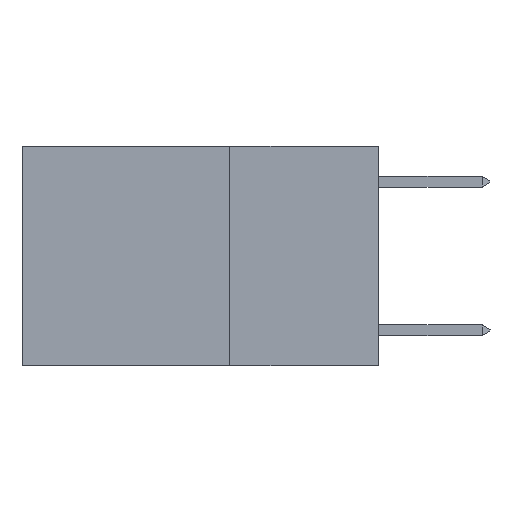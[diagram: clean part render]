
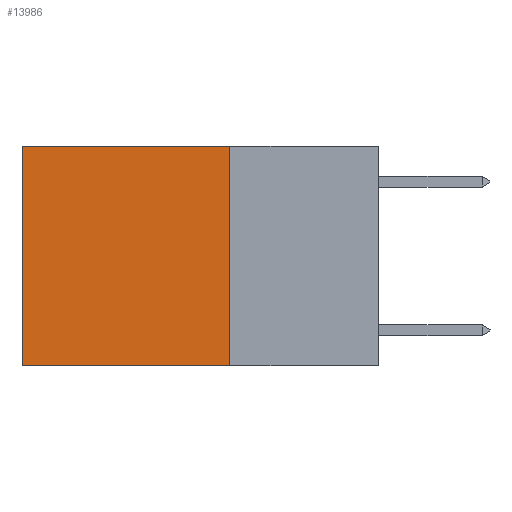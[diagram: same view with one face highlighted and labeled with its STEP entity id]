
A CAD part, left-side view. The second image highlights one B-rep face of the part: STEP entity #13986.
In plain terms, the highlighted planar face has unit normal (-1, 0, 0).
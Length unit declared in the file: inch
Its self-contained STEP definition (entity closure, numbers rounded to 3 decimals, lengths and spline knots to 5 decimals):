
#487 = CARTESIAN_POINT ( 'NONE',  ( 0.2625, 0.6, -0.37 ) ) ;
#1094 = ORIENTED_EDGE ( 'NONE', *, *, #10806, .T. ) ;
#1166 = CARTESIAN_POINT ( 'NONE',  ( 0.2625, 0.25, -0.37 ) ) ;
#2292 = VERTEX_POINT ( 'NONE', #487 ) ;
#2341 = LINE ( 'NONE', #16391, #19074 ) ;
#3539 = VECTOR ( 'NONE', #25348, 39.37008 ) ;
#3655 = CARTESIAN_POINT ( 'NONE',  ( 0.2625, 0.25, 0. ) ) ;
#5367 = VERTEX_POINT ( 'NONE', #16105 ) ;
#6586 = EDGE_LOOP ( 'NONE', ( #13706, #16342, #11652, #1094 ) ) ;
#7252 = DIRECTION ( 'NONE',  ( 0., 1., 0. ) ) ;
#10342 = CARTESIAN_POINT ( 'NONE',  ( 0.2625, 0.6, 0. ) ) ;
#10806 = EDGE_CURVE ( 'NONE', #26638, #20893, #2341, .T. ) ;
#11166 = CARTESIAN_POINT ( 'NONE',  ( 0.2625, 0.25, 0. ) ) ;
#11365 = PLANE ( 'NONE',  #17851 ) ;
#11652 = ORIENTED_EDGE ( 'NONE', *, *, #24643, .F. ) ;
#12000 = FACE_OUTER_BOUND ( 'NONE', #6586, .T. ) ;
#13599 = DIRECTION ( 'NONE',  ( 0., 0., -1. ) ) ;
#13706 = ORIENTED_EDGE ( 'NONE', *, *, #18353, .T. ) ;
#13986 = ADVANCED_FACE ( 'NONE', ( #12000 ), #11365, .F. ) ;
#15291 = CARTESIAN_POINT ( 'NONE',  ( 0.2625, 0.25, 0. ) ) ;
#15518 = DIRECTION ( 'NONE',  ( 1., 0., 0. ) ) ;
#16105 = CARTESIAN_POINT ( 'NONE',  ( 0.2625, 0.25, -0.37 ) ) ;
#16342 = ORIENTED_EDGE ( 'NONE', *, *, #23106, .F. ) ;
#16391 = CARTESIAN_POINT ( 'NONE',  ( 0.2625, 0.25, 0. ) ) ;
#16996 = DIRECTION ( 'NONE',  ( 0., 0., -1. ) ) ;
#17851 = AXIS2_PLACEMENT_3D ( 'NONE', #11166, #15518, #13599 ) ;
#18005 = VECTOR ( 'NONE', #18942, 39.37008 ) ;
#18329 = LINE ( 'NONE', #3655, #18005 ) ;
#18353 = EDGE_CURVE ( 'NONE', #20893, #2292, #23348, .T. ) ;
#18942 = DIRECTION ( 'NONE',  ( 0., 0., -1. ) ) ;
#19074 = VECTOR ( 'NONE', #7252, 39.37008 ) ;
#19749 = CARTESIAN_POINT ( 'NONE',  ( 0.2625, 0.6, 0. ) ) ;
#20893 = VERTEX_POINT ( 'NONE', #19749 ) ;
#21660 = VECTOR ( 'NONE', #16996, 39.37008 ) ;
#23106 = EDGE_CURVE ( 'NONE', #5367, #2292, #24046, .T. ) ;
#23348 = LINE ( 'NONE', #10342, #21660 ) ;
#24046 = LINE ( 'NONE', #1166, #3539 ) ;
#24643 = EDGE_CURVE ( 'NONE', #26638, #5367, #18329, .T. ) ;
#25348 = DIRECTION ( 'NONE',  ( 0., 1., 0. ) ) ;
#26638 = VERTEX_POINT ( 'NONE', #15291 ) ;
